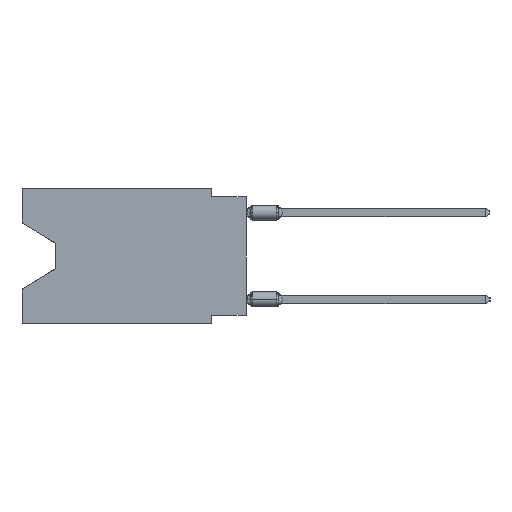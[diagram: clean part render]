
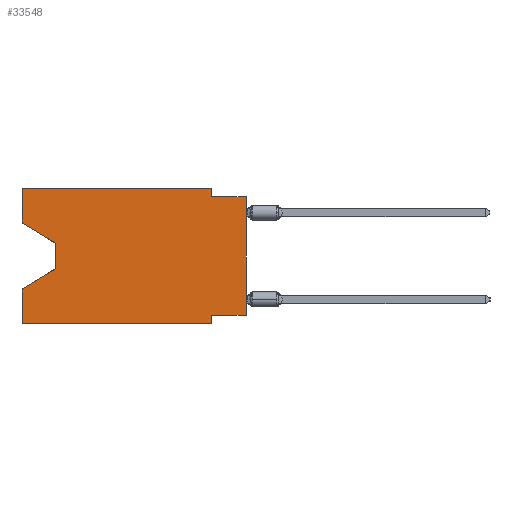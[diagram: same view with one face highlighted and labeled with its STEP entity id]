
A CAD part, left-side view. The second image highlights one B-rep face of the part: STEP entity #33548.
In plain terms, the highlighted planar face has unit normal (-1, 0, 0).
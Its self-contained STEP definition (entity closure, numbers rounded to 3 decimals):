
#53 = EDGE_CURVE ( 'NONE', #38210, #7233, #17725, .T. ) ;
#344 = EDGE_CURVE ( 'NONE', #7233, #3185, #37768, .T. ) ;
#629 = CARTESIAN_POINT ( 'NONE',  ( 0., 0., -9.271 ) ) ;
#1156 = VECTOR ( 'NONE', #16647, 1000. ) ;
#1196 = ORIENTED_EDGE ( 'NONE', *, *, #23448, .T. ) ;
#2414 = CARTESIAN_POINT ( 'NONE',  ( 0., 2.54, -9.271 ) ) ;
#3137 = CARTESIAN_POINT ( 'NONE',  ( 0., 2.54, 0. ) ) ;
#3185 = VERTEX_POINT ( 'NONE', #30271 ) ;
#3281 = VECTOR ( 'NONE', #7796, 1000. ) ;
#3520 = VERTEX_POINT ( 'NONE', #2414 ) ;
#3617 = CARTESIAN_POINT ( 'NONE',  ( 0., 16.383, 0. ) ) ;
#3651 = ORIENTED_EDGE ( 'NONE', *, *, #5025, .T. ) ;
#3840 = CARTESIAN_POINT ( 'NONE',  ( 0., 0., -0.635 ) ) ;
#3861 = LINE ( 'NONE', #15625, #30251 ) ;
#3894 = LINE ( 'NONE', #3137, #6488 ) ;
#4065 = DIRECTION ( 'NONE',  ( 0., -0.855, -0.519 ) ) ;
#4085 = EDGE_CURVE ( 'NONE', #22421, #3520, #15665, .T. ) ;
#4898 = CARTESIAN_POINT ( 'NONE',  ( 0., 13.97, -4.013 ) ) ;
#5025 = EDGE_CURVE ( 'NONE', #23855, #10818, #25000, .T. ) ;
#5334 = VECTOR ( 'NONE', #30725, 1000. ) ;
#5792 = VECTOR ( 'NONE', #28914, 1000. ) ;
#6488 = VECTOR ( 'NONE', #33277, 1000. ) ;
#6702 = LINE ( 'NONE', #12466, #31389 ) ;
#7156 = LINE ( 'NONE', #18924, #5334 ) ;
#7233 = VERTEX_POINT ( 'NONE', #25835 ) ;
#7796 = DIRECTION ( 'NONE',  ( 0., -1., 0. ) ) ;
#7806 = PLANE ( 'NONE',  #8971 ) ;
#8971 = AXIS2_PLACEMENT_3D ( 'NONE', #31173, #37354, #13176 ) ;
#9154 = DIRECTION ( 'NONE',  ( 0., 1., 0. ) ) ;
#9763 = ORIENTED_EDGE ( 'NONE', *, *, #21716, .T. ) ;
#10679 = FACE_OUTER_BOUND ( 'NONE', #21255, .T. ) ;
#10688 = VERTEX_POINT ( 'NONE', #14123 ) ;
#10818 = VERTEX_POINT ( 'NONE', #36794 ) ;
#12304 = VERTEX_POINT ( 'NONE', #30118 ) ;
#12466 = CARTESIAN_POINT ( 'NONE',  ( 0., 16.383, -9.906 ) ) ;
#12754 = VERTEX_POINT ( 'NONE', #30073 ) ;
#13047 = EDGE_CURVE ( 'NONE', #12754, #28225, #7156, .T. ) ;
#13176 = DIRECTION ( 'NONE',  ( 0., 0., -1. ) ) ;
#13428 = ORIENTED_EDGE ( 'NONE', *, *, #344, .F. ) ;
#13740 = LINE ( 'NONE', #18998, #1156 ) ;
#13912 = VECTOR ( 'NONE', #9154, 1000. ) ;
#14123 = CARTESIAN_POINT ( 'NONE',  ( 0., 2.54, -0.635 ) ) ;
#14148 = ORIENTED_EDGE ( 'NONE', *, *, #13047, .F. ) ;
#14298 = VECTOR ( 'NONE', #24290, 1000. ) ;
#15065 = ORIENTED_EDGE ( 'NONE', *, *, #24270, .F. ) ;
#15625 = CARTESIAN_POINT ( 'NONE',  ( 0., 16.383, -2.546 ) ) ;
#15665 = LINE ( 'NONE', #629, #13912 ) ;
#16176 = ORIENTED_EDGE ( 'NONE', *, *, #16192, .T. ) ;
#16192 = EDGE_CURVE ( 'NONE', #38210, #23855, #3861, .T. ) ;
#16647 = DIRECTION ( 'NONE',  ( 0., 0., 1. ) ) ;
#16694 = CARTESIAN_POINT ( 'NONE',  ( 0., 16.383, 0. ) ) ;
#17725 = LINE ( 'NONE', #3617, #14298 ) ;
#17998 = LINE ( 'NONE', #24192, #36125 ) ;
#18173 = VECTOR ( 'NONE', #25576, 1000. ) ;
#18924 = CARTESIAN_POINT ( 'NONE',  ( 0., 16.383, 0. ) ) ;
#18998 = CARTESIAN_POINT ( 'NONE',  ( 0., 0., 0. ) ) ;
#20203 = DIRECTION ( 'NONE',  ( 0., -1., 0. ) ) ;
#20675 = VERTEX_POINT ( 'NONE', #3840 ) ;
#20964 = ORIENTED_EDGE ( 'NONE', *, *, #36458, .T. ) ;
#21255 = EDGE_LOOP ( 'NONE', ( #16176, #3651, #20964, #14148, #1196, #15065, #27700, #9763, #26217, #37701, #13428, #21301 ) ) ;
#21301 = ORIENTED_EDGE ( 'NONE', *, *, #53, .F. ) ;
#21716 = EDGE_CURVE ( 'NONE', #22421, #20675, #13740, .T. ) ;
#22421 = VERTEX_POINT ( 'NONE', #36122 ) ;
#22856 = CARTESIAN_POINT ( 'NONE',  ( 0., 0., -0.635 ) ) ;
#23448 = EDGE_CURVE ( 'NONE', #12754, #12304, #6702, .T. ) ;
#23621 = VECTOR ( 'NONE', #20203, 1000. ) ;
#23744 = CARTESIAN_POINT ( 'NONE',  ( 0., 16.383, -7.36 ) ) ;
#23855 = VERTEX_POINT ( 'NONE', #30225 ) ;
#24192 = CARTESIAN_POINT ( 'NONE',  ( 0., 2.54, -9.906 ) ) ;
#24270 = EDGE_CURVE ( 'NONE', #3520, #12304, #17998, .T. ) ;
#24273 = DIRECTION ( 'NONE',  ( 0., -1., 0. ) ) ;
#24290 = DIRECTION ( 'NONE',  ( 0., 0., 1. ) ) ;
#25000 = LINE ( 'NONE', #4898, #18173 ) ;
#25576 = DIRECTION ( 'NONE',  ( 0., 0., -1. ) ) ;
#25835 = CARTESIAN_POINT ( 'NONE',  ( 0., 16.383, 0. ) ) ;
#26217 = ORIENTED_EDGE ( 'NONE', *, *, #35737, .F. ) ;
#27700 = ORIENTED_EDGE ( 'NONE', *, *, #4085, .F. ) ;
#28225 = VERTEX_POINT ( 'NONE', #23744 ) ;
#28656 = LINE ( 'NONE', #22856, #3281 ) ;
#28914 = DIRECTION ( 'NONE',  ( 0., 0.855, -0.519 ) ) ;
#29804 = DIRECTION ( 'NONE',  ( 0., 0., -1. ) ) ;
#30073 = CARTESIAN_POINT ( 'NONE',  ( 0., 16.383, -9.906 ) ) ;
#30118 = CARTESIAN_POINT ( 'NONE',  ( 0., 2.54, -9.906 ) ) ;
#30225 = CARTESIAN_POINT ( 'NONE',  ( 0., 13.97, -4.013 ) ) ;
#30251 = VECTOR ( 'NONE', #4065, 1000. ) ;
#30271 = CARTESIAN_POINT ( 'NONE',  ( 0., 2.54, 0. ) ) ;
#30725 = DIRECTION ( 'NONE',  ( 0., 0., 1. ) ) ;
#31173 = CARTESIAN_POINT ( 'NONE',  ( 0., 16.383, 0. ) ) ;
#31389 = VECTOR ( 'NONE', #24273, 1000. ) ;
#32158 = LINE ( 'NONE', #34500, #5792 ) ;
#33277 = DIRECTION ( 'NONE',  ( 0., 0., -1. ) ) ;
#33548 = ADVANCED_FACE ( 'NONE', ( #10679 ), #7806, .F. ) ;
#33819 = EDGE_CURVE ( 'NONE', #3185, #10688, #3894, .T. ) ;
#34500 = CARTESIAN_POINT ( 'NONE',  ( 0., 13.97, -5.893 ) ) ;
#34689 = CARTESIAN_POINT ( 'NONE',  ( 0., 16.383, -2.546 ) ) ;
#35737 = EDGE_CURVE ( 'NONE', #10688, #20675, #28656, .T. ) ;
#36122 = CARTESIAN_POINT ( 'NONE',  ( 0., 0., -9.271 ) ) ;
#36125 = VECTOR ( 'NONE', #29804, 1000. ) ;
#36458 = EDGE_CURVE ( 'NONE', #10818, #28225, #32158, .T. ) ;
#36794 = CARTESIAN_POINT ( 'NONE',  ( 0., 13.97, -5.893 ) ) ;
#37354 = DIRECTION ( 'NONE',  ( 1., 0., 0. ) ) ;
#37701 = ORIENTED_EDGE ( 'NONE', *, *, #33819, .F. ) ;
#37768 = LINE ( 'NONE', #16694, #23621 ) ;
#38210 = VERTEX_POINT ( 'NONE', #34689 ) ;
